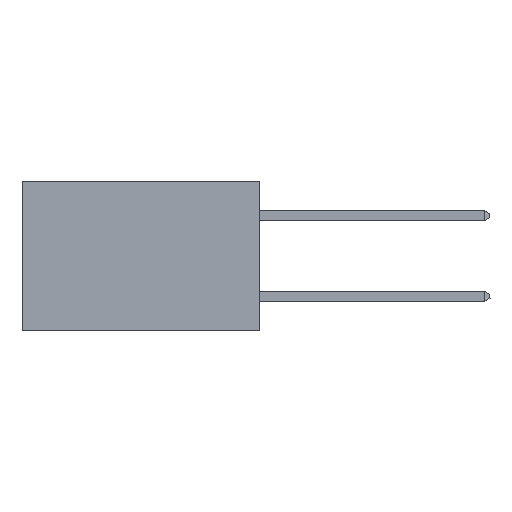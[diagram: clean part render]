
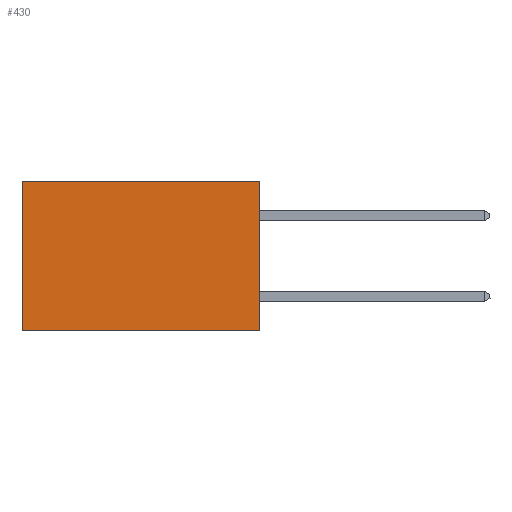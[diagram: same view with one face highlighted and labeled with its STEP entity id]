
A CAD part, left-side view. The second image highlights one B-rep face of the part: STEP entity #430.
In plain terms, the highlighted planar face has unit normal (-1, 0, 0).
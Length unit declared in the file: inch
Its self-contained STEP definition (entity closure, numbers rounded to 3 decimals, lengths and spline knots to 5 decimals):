
#211 = VECTOR ( 'NONE', #402, 39.37008 ) ;
#402 = DIRECTION ( 'NONE',  ( 0., 0., -1. ) ) ;
#430 = ADVANCED_FACE ( 'NONE', ( #8092 ), #1148, .F. ) ;
#770 = DIRECTION ( 'NONE',  ( 1., 0., 0. ) ) ;
#850 = ORIENTED_EDGE ( 'NONE', *, *, #12969, .T. ) ;
#1148 = PLANE ( 'NONE',  #8519 ) ;
#1178 = CARTESIAN_POINT ( 'NONE',  ( 0.277, 0., -0.37 ) ) ;
#1434 = LINE ( 'NONE', #4379, #12147 ) ;
#1485 = DIRECTION ( 'NONE',  ( 0., 1., 0. ) ) ;
#2201 = CARTESIAN_POINT ( 'NONE',  ( 0.277, 0., 0. ) ) ;
#2388 = EDGE_CURVE ( 'NONE', #10700, #6709, #13271, .T. ) ;
#2497 = EDGE_CURVE ( 'NONE', #3777, #7528, #11724, .T. ) ;
#3006 = CARTESIAN_POINT ( 'NONE',  ( 0.277, 0.59, 0. ) ) ;
#3777 = VERTEX_POINT ( 'NONE', #2201 ) ;
#3821 = LINE ( 'NONE', #10030, #6458 ) ;
#4300 = DIRECTION ( 'NONE',  ( 0., 1., 0. ) ) ;
#4379 = CARTESIAN_POINT ( 'NONE',  ( 0.277, 0., -0.37 ) ) ;
#4870 = CARTESIAN_POINT ( 'NONE',  ( 0.277, 0., -0.37 ) ) ;
#6458 = VECTOR ( 'NONE', #1485, 39.37008 ) ;
#6626 = CARTESIAN_POINT ( 'NONE',  ( 0.277, 0.59, -0.37 ) ) ;
#6709 = VERTEX_POINT ( 'NONE', #6626 ) ;
#6944 = EDGE_CURVE ( 'NONE', #7528, #6709, #1434, .T. ) ;
#7528 = VERTEX_POINT ( 'NONE', #13531 ) ;
#7857 = DIRECTION ( 'NONE',  ( 0., 0., -1. ) ) ;
#7881 = VECTOR ( 'NONE', #7857, 39.37008 ) ;
#8092 = FACE_OUTER_BOUND ( 'NONE', #12984, .T. ) ;
#8519 = AXIS2_PLACEMENT_3D ( 'NONE', #1178, #770, #9968 ) ;
#9968 = DIRECTION ( 'NONE',  ( 0., 0., -1. ) ) ;
#10030 = CARTESIAN_POINT ( 'NONE',  ( 0.277, 0., 0. ) ) ;
#10700 = VERTEX_POINT ( 'NONE', #3006 ) ;
#10933 = CARTESIAN_POINT ( 'NONE',  ( 0.277, 0.59, -0.37 ) ) ;
#11381 = ORIENTED_EDGE ( 'NONE', *, *, #6944, .F. ) ;
#11532 = ORIENTED_EDGE ( 'NONE', *, *, #2497, .F. ) ;
#11724 = LINE ( 'NONE', #4870, #211 ) ;
#11999 = ORIENTED_EDGE ( 'NONE', *, *, #2388, .T. ) ;
#12147 = VECTOR ( 'NONE', #4300, 39.37008 ) ;
#12969 = EDGE_CURVE ( 'NONE', #3777, #10700, #3821, .T. ) ;
#12984 = EDGE_LOOP ( 'NONE', ( #11999, #11381, #11532, #850 ) ) ;
#13271 = LINE ( 'NONE', #10933, #7881 ) ;
#13531 = CARTESIAN_POINT ( 'NONE',  ( 0.277, 0., -0.37 ) ) ;
